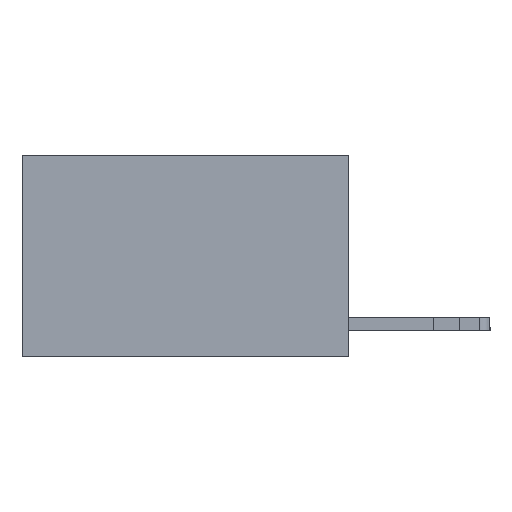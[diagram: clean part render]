
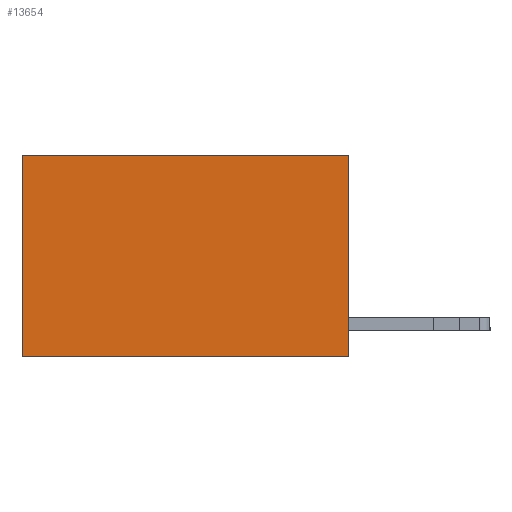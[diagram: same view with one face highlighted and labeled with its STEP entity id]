
A CAD part, left-side view. The second image highlights one B-rep face of the part: STEP entity #13654.
In plain terms, the highlighted planar face has unit normal (-1, 0, 0).
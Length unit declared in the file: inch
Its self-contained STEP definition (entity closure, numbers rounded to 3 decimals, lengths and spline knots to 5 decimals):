
#1158 = EDGE_CURVE ( 'NONE', #2397, #14396, #1164, .T. ) ;
#1164 = LINE ( 'NONE', #9293, #10039 ) ;
#1850 = DIRECTION ( 'NONE',  ( 0., 0., -1. ) ) ;
#2397 = VERTEX_POINT ( 'NONE', #21119 ) ;
#2587 = DIRECTION ( 'NONE',  ( 1., 0., 0. ) ) ;
#2958 = CARTESIAN_POINT ( 'NONE',  ( 0.2625, 0., -0.37 ) ) ;
#4568 = DIRECTION ( 'NONE',  ( 0., 1., 0. ) ) ;
#5991 = CARTESIAN_POINT ( 'NONE',  ( 0.2625, 0., 0. ) ) ;
#6264 = VECTOR ( 'NONE', #1850, 39.37008 ) ;
#6870 = VECTOR ( 'NONE', #13138, 39.37008 ) ;
#7480 = CARTESIAN_POINT ( 'NONE',  ( 0.2625, 0., 0. ) ) ;
#8383 = LINE ( 'NONE', #5991, #6264 ) ;
#8718 = EDGE_CURVE ( 'NONE', #25881, #12325, #11208, .T. ) ;
#9293 = CARTESIAN_POINT ( 'NONE',  ( 0.2625, 0., 0. ) ) ;
#10039 = VECTOR ( 'NONE', #17389, 39.37008 ) ;
#10834 = EDGE_CURVE ( 'NONE', #2397, #25881, #8383, .T. ) ;
#11208 = LINE ( 'NONE', #2958, #17921 ) ;
#12325 = VERTEX_POINT ( 'NONE', #13051 ) ;
#13051 = CARTESIAN_POINT ( 'NONE',  ( 0.2625, 0.6, -0.37 ) ) ;
#13138 = DIRECTION ( 'NONE',  ( 0., 0., -1. ) ) ;
#13280 = ORIENTED_EDGE ( 'NONE', *, *, #8718, .F. ) ;
#13654 = ADVANCED_FACE ( 'NONE', ( #25152 ), #25634, .F. ) ;
#14014 = ORIENTED_EDGE ( 'NONE', *, *, #16719, .T. ) ;
#14396 = VERTEX_POINT ( 'NONE', #16733 ) ;
#14999 = CARTESIAN_POINT ( 'NONE',  ( 0.2625, 0.6, 0. ) ) ;
#15762 = ORIENTED_EDGE ( 'NONE', *, *, #10834, .F. ) ;
#16719 = EDGE_CURVE ( 'NONE', #14396, #12325, #19246, .T. ) ;
#16733 = CARTESIAN_POINT ( 'NONE',  ( 0.2625, 0.6, 0. ) ) ;
#16909 = AXIS2_PLACEMENT_3D ( 'NONE', #7480, #2587, #23651 ) ;
#17389 = DIRECTION ( 'NONE',  ( 0., 1., 0. ) ) ;
#17597 = EDGE_LOOP ( 'NONE', ( #14014, #13280, #15762, #22142 ) ) ;
#17921 = VECTOR ( 'NONE', #4568, 39.37008 ) ;
#19246 = LINE ( 'NONE', #14999, #6870 ) ;
#21119 = CARTESIAN_POINT ( 'NONE',  ( 0.2625, 0., 0. ) ) ;
#22142 = ORIENTED_EDGE ( 'NONE', *, *, #1158, .T. ) ;
#23651 = DIRECTION ( 'NONE',  ( 0., 0., -1. ) ) ;
#23728 = CARTESIAN_POINT ( 'NONE',  ( 0.2625, 0., -0.37 ) ) ;
#25152 = FACE_OUTER_BOUND ( 'NONE', #17597, .T. ) ;
#25634 = PLANE ( 'NONE',  #16909 ) ;
#25881 = VERTEX_POINT ( 'NONE', #23728 ) ;
